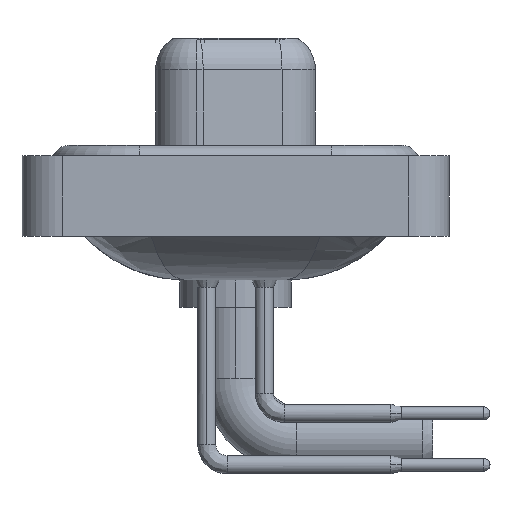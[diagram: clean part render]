
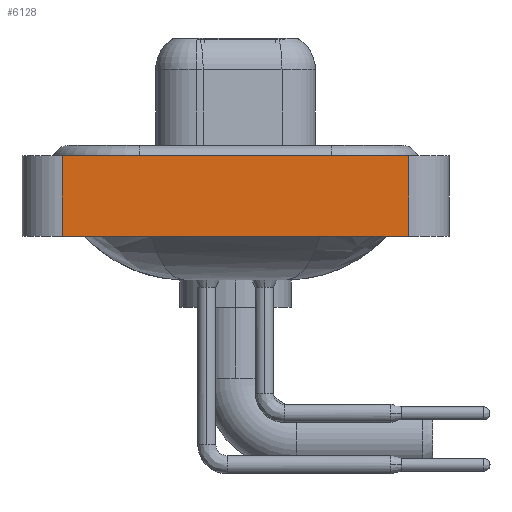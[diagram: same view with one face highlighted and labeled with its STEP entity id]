
A CAD part, left-side view. The second image highlights one B-rep face of the part: STEP entity #6128.
In plain terms, the highlighted planar face has unit normal (-1, 0, 0).
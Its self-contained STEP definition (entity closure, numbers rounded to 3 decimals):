
#1199 = LINE ( 'NONE', #9327, #7307 ) ;
#2496 = VECTOR ( 'NONE', #4212, 1000. ) ;
#4117 = ORIENTED_EDGE ( 'NONE', *, *, #24301, .F. ) ;
#4212 = DIRECTION ( 'NONE',  ( 0., 0., 1. ) ) ;
#5744 = CARTESIAN_POINT ( 'NONE',  ( -7.35, -8.55, 0.4 ) ) ;
#6128 = ADVANCED_FACE ( 'NONE', ( #14644 ), #14507, .T. ) ;
#6358 = CARTESIAN_POINT ( 'NONE',  ( -7.35, 8.55, -3.6 ) ) ;
#6368 = EDGE_LOOP ( 'NONE', ( #18687, #4117, #8519, #13894 ) ) ;
#7307 = VECTOR ( 'NONE', #17482, 1000. ) ;
#7585 = VECTOR ( 'NONE', #22792, 1000. ) ;
#8519 = ORIENTED_EDGE ( 'NONE', *, *, #19187, .F. ) ;
#8751 = DIRECTION ( 'NONE',  ( -1., 0., 0. ) ) ;
#9327 = CARTESIAN_POINT ( 'NONE',  ( -7.35, -8.55, -3.6 ) ) ;
#9430 = LINE ( 'NONE', #17585, #26117 ) ;
#11663 = VERTEX_POINT ( 'NONE', #11928 ) ;
#11766 = CARTESIAN_POINT ( 'NONE',  ( -7.35, 8.55, 0.4 ) ) ;
#11928 = CARTESIAN_POINT ( 'NONE',  ( -7.35, 8.55, -3.6 ) ) ;
#12477 = CARTESIAN_POINT ( 'NONE',  ( -7.35, -8.55, -3.6 ) ) ;
#13894 = ORIENTED_EDGE ( 'NONE', *, *, #23387, .T. ) ;
#13999 = VERTEX_POINT ( 'NONE', #5744 ) ;
#14368 = DIRECTION ( 'NONE',  ( 0., 0., 1. ) ) ;
#14507 = PLANE ( 'NONE',  #14705 ) ;
#14644 = FACE_OUTER_BOUND ( 'NONE', #6368, .T. ) ;
#14701 = CARTESIAN_POINT ( 'NONE',  ( -7.35, -8.55, -3.6 ) ) ;
#14705 = AXIS2_PLACEMENT_3D ( 'NONE', #24636, #8751, #14368 ) ;
#15155 = EDGE_CURVE ( 'NONE', #23148, #13999, #18765, .T. ) ;
#16095 = DIRECTION ( 'NONE',  ( 0., -1., 0. ) ) ;
#17482 = DIRECTION ( 'NONE',  ( 0., -1., 0. ) ) ;
#17585 = CARTESIAN_POINT ( 'NONE',  ( -7.35, -8.55, 0.4 ) ) ;
#18372 = LINE ( 'NONE', #6358, #7585 ) ;
#18687 = ORIENTED_EDGE ( 'NONE', *, *, #15155, .T. ) ;
#18765 = LINE ( 'NONE', #12477, #2496 ) ;
#19187 = EDGE_CURVE ( 'NONE', #11663, #24759, #18372, .T. ) ;
#22792 = DIRECTION ( 'NONE',  ( 0., 0., 1. ) ) ;
#23148 = VERTEX_POINT ( 'NONE', #14701 ) ;
#23387 = EDGE_CURVE ( 'NONE', #11663, #23148, #1199, .T. ) ;
#24301 = EDGE_CURVE ( 'NONE', #24759, #13999, #9430, .T. ) ;
#24636 = CARTESIAN_POINT ( 'NONE',  ( -7.35, -8.55, -3.6 ) ) ;
#24759 = VERTEX_POINT ( 'NONE', #11766 ) ;
#26117 = VECTOR ( 'NONE', #16095, 1000. ) ;
